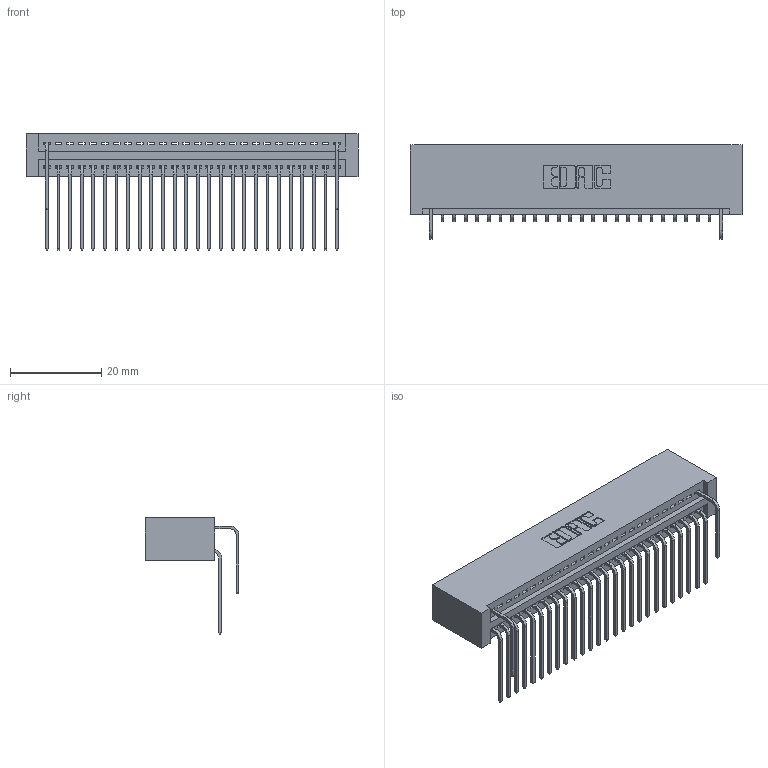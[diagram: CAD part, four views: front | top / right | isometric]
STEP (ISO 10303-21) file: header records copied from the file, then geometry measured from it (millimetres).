
FILE_DESCRIPTION (( 'STEP AP203' ), '1' );
FILE_NAME ('345-052-559-201.STEP', '2018-09-23T00:39:22', ( '' ), ( '' ), 'SwSTEP 2.0', 'SolidWorks 2016', '' );
FILE_SCHEMA (( 'CONFIG_CONTROL_DESIGN' ));
Length unit declared in the file: inch
Products named in the file (4): 345 Part_No Mounting Lugs; 345-292-001_558 559 Tail - 1; 345-292-001_559 Tail - 2; 345-052-559-201
Assembly tree (29 placements, depth 2):
  345-052-559-201
    345 Part_No Mounting Lugs
    345-292-001_558 559 Tail - 1  x26
    345-292-001_559 Tail - 2  x2
Bounding box: 72.64 x 20.56 x 25.53 mm (x, y, z)
Volume: 7469.3 mm3; surface area: 10568.5 mm2
Topology: 29 solids, 29 shells, 1766 faces, 5305 edges, 3498 vertices
Faces by surface type: plane 1224, cylinder 542
Entity records: 23161 total; most frequent: CARTESIAN_POINT 4047, ORIENTED_EDGE 3954, DIRECTION 3529, EDGE_CURVE 1977, LINE 1709, VECTOR 1709, VERTEX_POINT 1314, AXIS2_PLACEMENT_3D 910
